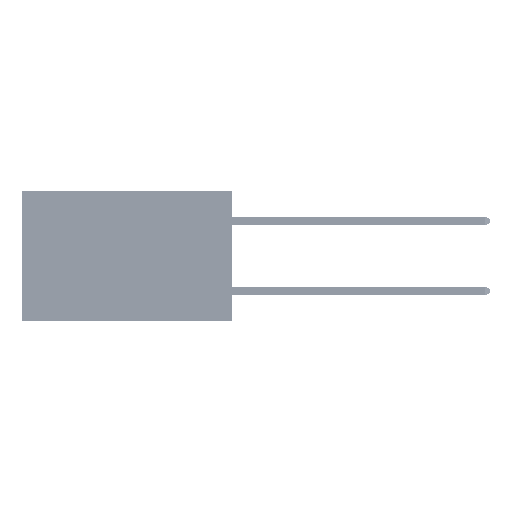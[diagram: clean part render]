
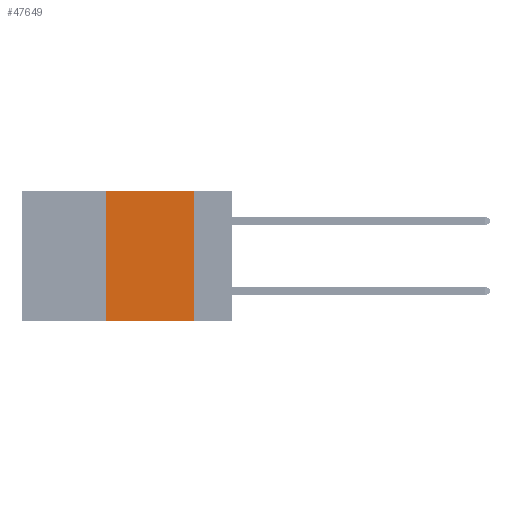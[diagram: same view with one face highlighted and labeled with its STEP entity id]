
A CAD part, left-side view. The second image highlights one B-rep face of the part: STEP entity #47649.
In plain terms, the highlighted planar face has unit normal (-1, 0, 0).
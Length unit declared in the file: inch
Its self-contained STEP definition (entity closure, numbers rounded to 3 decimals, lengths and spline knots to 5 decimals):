
#1695 = CARTESIAN_POINT ( 'NONE',  ( 0., 0.36, 0. ) ) ;
#3175 = EDGE_CURVE ( 'NONE', #17328, #7469, #22073, .T. ) ;
#4557 = ORIENTED_EDGE ( 'NONE', *, *, #10375, .F. ) ;
#4937 = VECTOR ( 'NONE', #41500, 39.37008 ) ;
#5526 = CARTESIAN_POINT ( 'NONE',  ( 0., 0.6, 0. ) ) ;
#6713 = VECTOR ( 'NONE', #17742, 39.37008 ) ;
#7469 = VERTEX_POINT ( 'NONE', #24268 ) ;
#7761 = DIRECTION ( 'NONE',  ( 0., -1., 0. ) ) ;
#8108 = AXIS2_PLACEMENT_3D ( 'NONE', #42415, #34045, #38246 ) ;
#10375 = EDGE_CURVE ( 'NONE', #21764, #7469, #12905, .T. ) ;
#10763 = ORIENTED_EDGE ( 'NONE', *, *, #15220, .F. ) ;
#11249 = FACE_OUTER_BOUND ( 'NONE', #29494, .T. ) ;
#12905 = LINE ( 'NONE', #22541, #31692 ) ;
#14139 = PLANE ( 'NONE',  #8108 ) ;
#15220 = EDGE_CURVE ( 'NONE', #17328, #38182, #22939, .T. ) ;
#17328 = VERTEX_POINT ( 'NONE', #49023 ) ;
#17562 = CARTESIAN_POINT ( 'NONE',  ( 0., 0.36, 0. ) ) ;
#17742 = DIRECTION ( 'NONE',  ( 0., 0., 1. ) ) ;
#19265 = EDGE_CURVE ( 'NONE', #38182, #21764, #42462, .T. ) ;
#21764 = VERTEX_POINT ( 'NONE', #51623 ) ;
#22073 = LINE ( 'NONE', #43384, #27690 ) ;
#22541 = CARTESIAN_POINT ( 'NONE',  ( 0., 0.11, 0. ) ) ;
#22939 = LINE ( 'NONE', #17562, #6713 ) ;
#24268 = CARTESIAN_POINT ( 'NONE',  ( 0., 0.11, -0.37 ) ) ;
#27249 = ORIENTED_EDGE ( 'NONE', *, *, #19265, .F. ) ;
#27690 = VECTOR ( 'NONE', #7761, 39.37008 ) ;
#29494 = EDGE_LOOP ( 'NONE', ( #4557, #27249, #10763, #41029 ) ) ;
#31692 = VECTOR ( 'NONE', #38458, 39.37008 ) ;
#34045 = DIRECTION ( 'NONE',  ( 1., 0., 0. ) ) ;
#38182 = VERTEX_POINT ( 'NONE', #1695 ) ;
#38246 = DIRECTION ( 'NONE',  ( 0., 0., -1. ) ) ;
#38458 = DIRECTION ( 'NONE',  ( 0., 0., -1. ) ) ;
#41029 = ORIENTED_EDGE ( 'NONE', *, *, #3175, .T. ) ;
#41500 = DIRECTION ( 'NONE',  ( 0., -1., 0. ) ) ;
#42415 = CARTESIAN_POINT ( 'NONE',  ( 0., 0.6, 0. ) ) ;
#42462 = LINE ( 'NONE', #5526, #4937 ) ;
#43384 = CARTESIAN_POINT ( 'NONE',  ( 0., 0.6, -0.37 ) ) ;
#47649 = ADVANCED_FACE ( 'NONE', ( #11249 ), #14139, .F. ) ;
#49023 = CARTESIAN_POINT ( 'NONE',  ( 0., 0.36, -0.37 ) ) ;
#51623 = CARTESIAN_POINT ( 'NONE',  ( 0., 0.11, 0. ) ) ;
